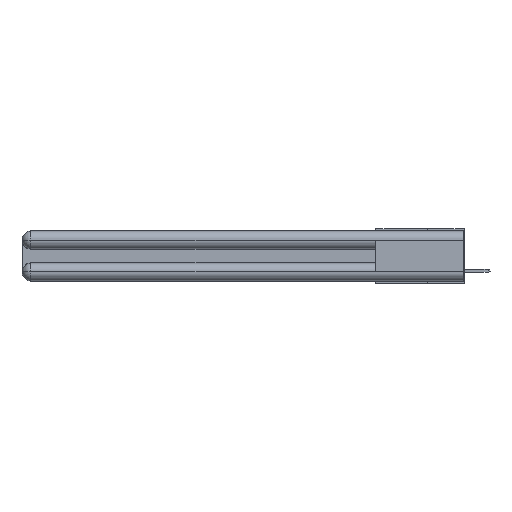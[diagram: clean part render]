
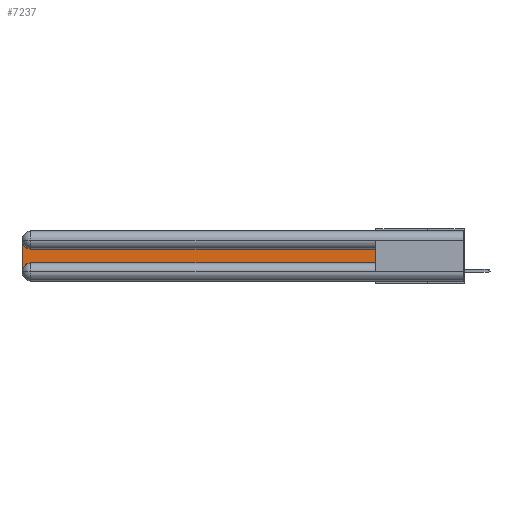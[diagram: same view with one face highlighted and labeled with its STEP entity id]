
A CAD part, left-side view. The second image highlights one B-rep face of the part: STEP entity #7237.
In plain terms, the highlighted planar face has unit normal (-1, 0, 0).
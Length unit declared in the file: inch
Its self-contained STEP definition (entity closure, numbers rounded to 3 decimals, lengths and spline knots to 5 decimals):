
#854 = DIRECTION ( 'NONE',  ( 0., 0., -1. ) ) ;
#1031 = EDGE_CURVE ( 'NONE', #13816, #29193, #32632, .T. ) ;
#2901 = CIRCLE ( 'NONE', #22639, 0.06 ) ;
#3215 = VECTOR ( 'NONE', #33707, 39.37008 ) ;
#3752 = VERTEX_POINT ( 'NONE', #24537 ) ;
#3901 = DIRECTION ( 'NONE',  ( 1., 0., 0. ) ) ;
#4108 = DIRECTION ( 'NONE',  ( 0., 0., -1. ) ) ;
#6034 = EDGE_CURVE ( 'NONE', #6943, #21633, #24490, .T. ) ;
#6342 = DIRECTION ( 'NONE',  ( 0., 1., 0. ) ) ;
#6547 = CARTESIAN_POINT ( 'NONE',  ( 0.075, 3., -0.2775 ) ) ;
#6835 = DIRECTION ( 'NONE',  ( 1., 0., 0. ) ) ;
#6943 = VERTEX_POINT ( 'NONE', #15245 ) ;
#7237 = ADVANCED_FACE ( 'NONE', ( #24538 ), #32820, .F. ) ;
#7536 = EDGE_CURVE ( 'NONE', #12126, #3752, #13250, .T. ) ;
#7974 = CARTESIAN_POINT ( 'NONE',  ( 0.075, 3., -0.0625 ) ) ;
#8601 = CARTESIAN_POINT ( 'NONE',  ( 0.075, 3., -0.1225 ) ) ;
#9297 = DIRECTION ( 'NONE',  ( 0., 0., -1. ) ) ;
#10507 = ORIENTED_EDGE ( 'NONE', *, *, #21535, .T. ) ;
#10631 = CARTESIAN_POINT ( 'NONE',  ( 0.075, 0.6, -0.2175 ) ) ;
#12126 = VERTEX_POINT ( 'NONE', #13588 ) ;
#12135 = CARTESIAN_POINT ( 'NONE',  ( 0.075, 0.6, -0.2175 ) ) ;
#13250 = LINE ( 'NONE', #16710, #14508 ) ;
#13588 = CARTESIAN_POINT ( 'NONE',  ( 0.075, 0.6, -0.1225 ) ) ;
#13816 = VERTEX_POINT ( 'NONE', #7974 ) ;
#14284 = ORIENTED_EDGE ( 'NONE', *, *, #7536, .T. ) ;
#14508 = VECTOR ( 'NONE', #6342, 39.37008 ) ;
#14967 = DIRECTION ( 'NONE',  ( 0., 0., -1. ) ) ;
#15245 = CARTESIAN_POINT ( 'NONE',  ( 0.075, 2.94, -0.2175 ) ) ;
#16710 = CARTESIAN_POINT ( 'NONE',  ( 0.075, 0.6, -0.1225 ) ) ;
#17483 = ORIENTED_EDGE ( 'NONE', *, *, #21374, .T. ) ;
#19813 = CARTESIAN_POINT ( 'NONE',  ( 0.075, 3., -0.2175 ) ) ;
#19989 = EDGE_CURVE ( 'NONE', #21633, #12126, #25127, .T. ) ;
#21250 = ORIENTED_EDGE ( 'NONE', *, *, #19989, .T. ) ;
#21374 = EDGE_CURVE ( 'NONE', #3752, #13816, #2901, .T. ) ;
#21535 = EDGE_CURVE ( 'NONE', #29193, #6943, #30885, .T. ) ;
#21633 = VERTEX_POINT ( 'NONE', #10631 ) ;
#22639 = AXIS2_PLACEMENT_3D ( 'NONE', #24984, #3901, #9297 ) ;
#24490 = LINE ( 'NONE', #12135, #3215 ) ;
#24537 = CARTESIAN_POINT ( 'NONE',  ( 0.075, 2.94, -0.1225 ) ) ;
#24538 = FACE_OUTER_BOUND ( 'NONE', #24539, .T. ) ;
#24539 = EDGE_LOOP ( 'NONE', ( #14284, #17483, #32251, #10507, #27036, #21250 ) ) ;
#24984 = CARTESIAN_POINT ( 'NONE',  ( 0.075, 2.94, -0.0625 ) ) ;
#25127 = LINE ( 'NONE', #33186, #28050 ) ;
#25349 = DIRECTION ( 'NONE',  ( 0., 0., 1. ) ) ;
#25484 = AXIS2_PLACEMENT_3D ( 'NONE', #8601, #27209, #854 ) ;
#25556 = CARTESIAN_POINT ( 'NONE',  ( 0.075, 2.94, -0.2775 ) ) ;
#27036 = ORIENTED_EDGE ( 'NONE', *, *, #6034, .T. ) ;
#27209 = DIRECTION ( 'NONE',  ( 1., 0., 0. ) ) ;
#28050 = VECTOR ( 'NONE', #25349, 39.37008 ) ;
#29193 = VERTEX_POINT ( 'NONE', #6547 ) ;
#29312 = VECTOR ( 'NONE', #4108, 39.37008 ) ;
#30885 = CIRCLE ( 'NONE', #32476, 0.06 ) ;
#32251 = ORIENTED_EDGE ( 'NONE', *, *, #1031, .T. ) ;
#32476 = AXIS2_PLACEMENT_3D ( 'NONE', #25556, #6835, #14967 ) ;
#32632 = LINE ( 'NONE', #19813, #29312 ) ;
#32820 = PLANE ( 'NONE',  #25484 ) ;
#33186 = CARTESIAN_POINT ( 'NONE',  ( 0.075, 0.6, -0.2175 ) ) ;
#33707 = DIRECTION ( 'NONE',  ( 0., -1., 0. ) ) ;
